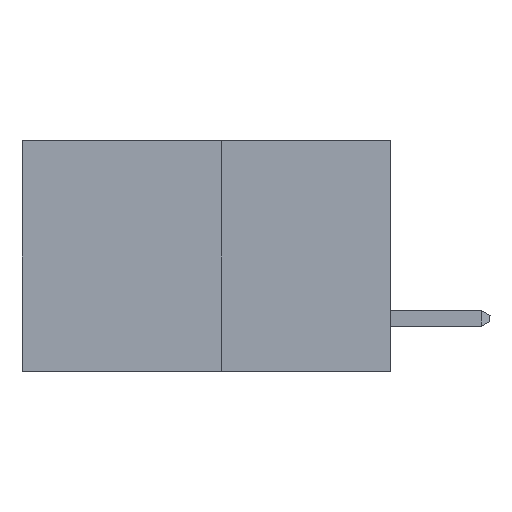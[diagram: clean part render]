
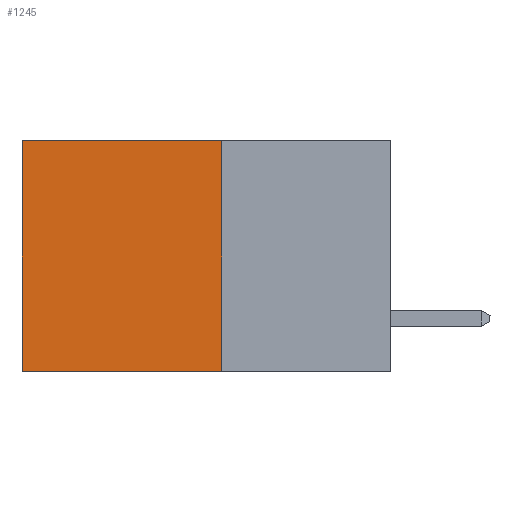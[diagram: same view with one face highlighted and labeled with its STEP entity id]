
A CAD part, left-side view. The second image highlights one B-rep face of the part: STEP entity #1245.
In plain terms, the highlighted planar face has unit normal (-1, 0, 0).
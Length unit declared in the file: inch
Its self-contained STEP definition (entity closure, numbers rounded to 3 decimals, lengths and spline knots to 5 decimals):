
#8 = EDGE_CURVE ( 'NONE', #8791, #8644, #9822, .T. ) ;
#93 = EDGE_CURVE ( 'NONE', #960, #8644, #6168, .T. ) ;
#401 = LINE ( 'NONE', #2475, #4795 ) ;
#895 = AXIS2_PLACEMENT_3D ( 'NONE', #10010, #4316, #10861 ) ;
#948 = CARTESIAN_POINT ( 'NONE',  ( 0.277, 0.59, 0. ) ) ;
#960 = VERTEX_POINT ( 'NONE', #948 ) ;
#1245 = ADVANCED_FACE ( 'NONE', ( #3626 ), #4339, .F. ) ;
#1277 = EDGE_CURVE ( 'NONE', #5326, #8791, #3356, .T. ) ;
#2475 = CARTESIAN_POINT ( 'NONE',  ( 0.277, 0.27, 0. ) ) ;
#2927 = VECTOR ( 'NONE', #8770, 39.37008 ) ;
#3356 = LINE ( 'NONE', #3523, #7415 ) ;
#3430 = DIRECTION ( 'NONE',  ( 0., 1., 0. ) ) ;
#3523 = CARTESIAN_POINT ( 'NONE',  ( 0.277, 0.27, -0.37 ) ) ;
#3626 = FACE_OUTER_BOUND ( 'NONE', #6915, .T. ) ;
#4316 = DIRECTION ( 'NONE',  ( 1., 0., 0. ) ) ;
#4339 = PLANE ( 'NONE',  #895 ) ;
#4427 = VECTOR ( 'NONE', #10151, 39.37008 ) ;
#4795 = VECTOR ( 'NONE', #3430, 39.37008 ) ;
#5137 = CARTESIAN_POINT ( 'NONE',  ( 0.277, 0.27, 0. ) ) ;
#5218 = ORIENTED_EDGE ( 'NONE', *, *, #93, .T. ) ;
#5326 = VERTEX_POINT ( 'NONE', #5137 ) ;
#5524 = ORIENTED_EDGE ( 'NONE', *, *, #8, .F. ) ;
#5896 = ORIENTED_EDGE ( 'NONE', *, *, #1277, .F. ) ;
#5986 = ORIENTED_EDGE ( 'NONE', *, *, #10765, .T. ) ;
#6168 = LINE ( 'NONE', #11401, #4427 ) ;
#6394 = CARTESIAN_POINT ( 'NONE',  ( 0.277, 0.27, -0.37 ) ) ;
#6915 = EDGE_LOOP ( 'NONE', ( #5218, #5524, #5896, #5986 ) ) ;
#7415 = VECTOR ( 'NONE', #9027, 39.37008 ) ;
#8644 = VERTEX_POINT ( 'NONE', #10364 ) ;
#8770 = DIRECTION ( 'NONE',  ( 0., 1., 0. ) ) ;
#8791 = VERTEX_POINT ( 'NONE', #6394 ) ;
#9027 = DIRECTION ( 'NONE',  ( 0., 0., -1. ) ) ;
#9822 = LINE ( 'NONE', #10169, #2927 ) ;
#10010 = CARTESIAN_POINT ( 'NONE',  ( 0.277, 0.27, -0.37 ) ) ;
#10151 = DIRECTION ( 'NONE',  ( 0., 0., -1. ) ) ;
#10169 = CARTESIAN_POINT ( 'NONE',  ( 0.277, 0.27, -0.37 ) ) ;
#10364 = CARTESIAN_POINT ( 'NONE',  ( 0.277, 0.59, -0.37 ) ) ;
#10765 = EDGE_CURVE ( 'NONE', #5326, #960, #401, .T. ) ;
#10861 = DIRECTION ( 'NONE',  ( 0., 0., -1. ) ) ;
#11401 = CARTESIAN_POINT ( 'NONE',  ( 0.277, 0.59, -0.37 ) ) ;
